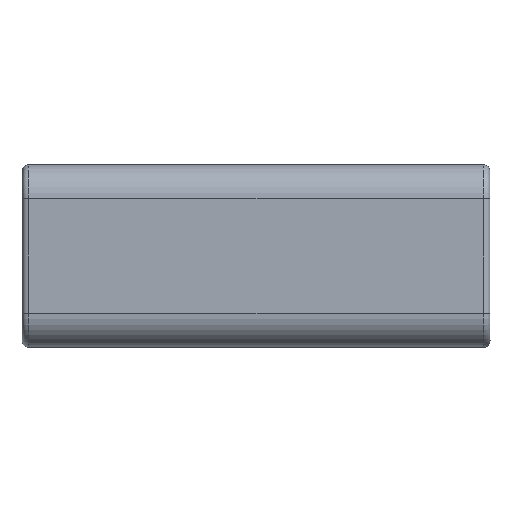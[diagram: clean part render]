
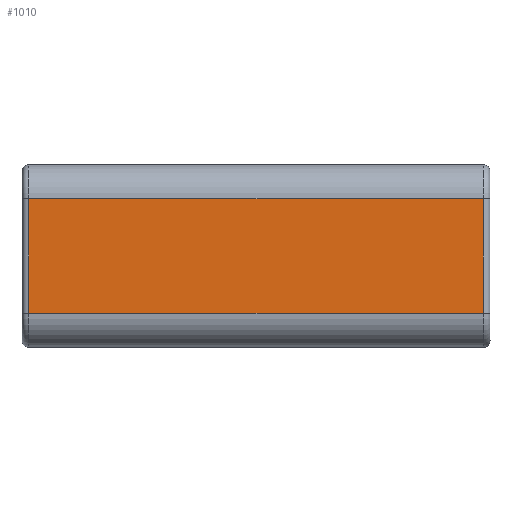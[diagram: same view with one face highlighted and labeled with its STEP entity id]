
A CAD part, front view. The second image highlights one B-rep face of the part: STEP entity #1010.
In plain terms, the highlighted planar face has unit normal (0, -1, 0).
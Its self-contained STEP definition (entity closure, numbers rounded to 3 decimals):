
#42=PLANE('',#1111);
#76=FACE_OUTER_BOUND('',#140,.T.);
#140=EDGE_LOOP('',(#733,#734,#735,#736));
#212=LINE('',#1733,#292);
#214=LINE('',#1742,#294);
#216=LINE('',#1748,#296);
#217=LINE('',#1749,#297);
#292=VECTOR('',#1284,10.);
#294=VECTOR('',#1296,10.);
#296=VECTOR('',#1302,10.);
#297=VECTOR('',#1303,10.);
#444=VERTEX_POINT('',#1727);
#445=VERTEX_POINT('',#1731);
#447=VERTEX_POINT('',#1741);
#449=VERTEX_POINT('',#1747);
#548=EDGE_CURVE('',#444,#445,#212,.T.);
#552=EDGE_CURVE('',#445,#447,#214,.T.);
#555=EDGE_CURVE('',#449,#444,#216,.T.);
#556=EDGE_CURVE('',#447,#449,#217,.T.);
#733=ORIENTED_EDGE('',*,*,#555,.F.);
#734=ORIENTED_EDGE('',*,*,#556,.F.);
#735=ORIENTED_EDGE('',*,*,#552,.F.);
#736=ORIENTED_EDGE('',*,*,#548,.F.);
#1010=ADVANCED_FACE('',(#76),#42,.T.);
#1111=AXIS2_PLACEMENT_3D('',#1746,#1300,#1301);
#1284=DIRECTION('',(0.,0.,-1.));
#1296=DIRECTION('',(-1.,0.,0.));
#1300=DIRECTION('center_axis',(0.,-1.,
0.));
#1301=DIRECTION('ref_axis',(0.,0.,1.));
#1302=DIRECTION('',(1.,0.,0.));
#1303=DIRECTION('',(0.,0.,1.));
#1727=CARTESIAN_POINT('',(182.918,-36.854,8.367));
#1731=CARTESIAN_POINT('',(182.918,-36.854,-8.565));
#1733=CARTESIAN_POINT('',(182.918,-36.854,-6.832));
#1741=CARTESIAN_POINT('',(115.95,-36.854,-8.565));
#1742=CARTESIAN_POINT('',(183.918,-36.854,-8.565));
#1746=CARTESIAN_POINT('Origin',(223.918,-36.854,-13.565));
#1747=CARTESIAN_POINT('',(115.95,-36.854,8.367));
#1748=CARTESIAN_POINT('',(183.918,-36.854,8.367));
#1749=CARTESIAN_POINT('',(115.95,-36.854,-6.832));
